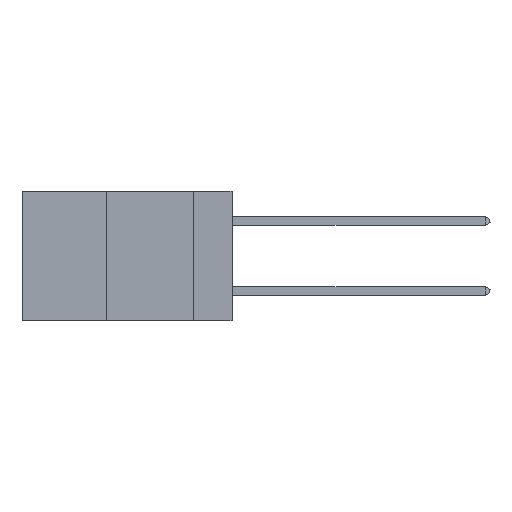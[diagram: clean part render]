
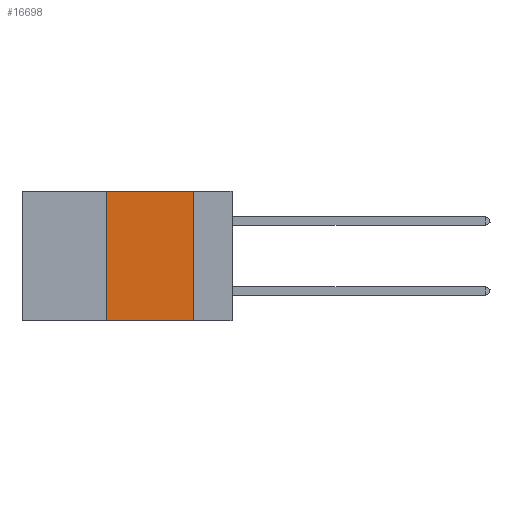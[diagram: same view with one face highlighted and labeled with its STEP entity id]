
A CAD part, left-side view. The second image highlights one B-rep face of the part: STEP entity #16698.
In plain terms, the highlighted planar face has unit normal (-1, 0, 0).
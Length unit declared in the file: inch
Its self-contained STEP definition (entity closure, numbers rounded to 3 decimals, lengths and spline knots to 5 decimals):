
#126 = VERTEX_POINT ( 'NONE', #13066 ) ;
#151 = LINE ( 'NONE', #2767, #1599 ) ;
#1599 = VECTOR ( 'NONE', #2745, 39.37008 ) ;
#2368 = VECTOR ( 'NONE', #10000, 39.37008 ) ;
#2745 = DIRECTION ( 'NONE',  ( 0., -1., 0. ) ) ;
#2767 = CARTESIAN_POINT ( 'NONE',  ( 0., 0.6, 0. ) ) ;
#3157 = CARTESIAN_POINT ( 'NONE',  ( 0., 0.36, 0. ) ) ;
#4890 = DIRECTION ( 'NONE',  ( 0., 0., -1. ) ) ;
#5109 = AXIS2_PLACEMENT_3D ( 'NONE', #5774, #8583, #13557 ) ;
#5685 = EDGE_CURVE ( 'NONE', #17000, #12538, #151, .T. ) ;
#5774 = CARTESIAN_POINT ( 'NONE',  ( 0., 0.6, 0. ) ) ;
#5812 = CARTESIAN_POINT ( 'NONE',  ( 0., 0.6, -0.37 ) ) ;
#5912 = ORIENTED_EDGE ( 'NONE', *, *, #5685, .F. ) ;
#6139 = LINE ( 'NONE', #5812, #2368 ) ;
#7488 = VERTEX_POINT ( 'NONE', #13101 ) ;
#7607 = LINE ( 'NONE', #10349, #17950 ) ;
#8424 = CARTESIAN_POINT ( 'NONE',  ( 0., 0.11, 0. ) ) ;
#8583 = DIRECTION ( 'NONE',  ( 1., 0., 0. ) ) ;
#8735 = EDGE_CURVE ( 'NONE', #12538, #126, #7607, .T. ) ;
#8835 = DIRECTION ( 'NONE',  ( 0., 0., 1. ) ) ;
#9533 = EDGE_LOOP ( 'NONE', ( #15918, #5912, #13139, #16035 ) ) ;
#9678 = LINE ( 'NONE', #3157, #15607 ) ;
#10000 = DIRECTION ( 'NONE',  ( 0., -1., 0. ) ) ;
#10349 = CARTESIAN_POINT ( 'NONE',  ( 0., 0.11, 0. ) ) ;
#10872 = EDGE_CURVE ( 'NONE', #7488, #17000, #9678, .T. ) ;
#12104 = FACE_OUTER_BOUND ( 'NONE', #9533, .T. ) ;
#12143 = CARTESIAN_POINT ( 'NONE',  ( 0., 0.36, 0. ) ) ;
#12538 = VERTEX_POINT ( 'NONE', #8424 ) ;
#13066 = CARTESIAN_POINT ( 'NONE',  ( 0., 0.11, -0.37 ) ) ;
#13101 = CARTESIAN_POINT ( 'NONE',  ( 0., 0.36, -0.37 ) ) ;
#13139 = ORIENTED_EDGE ( 'NONE', *, *, #10872, .F. ) ;
#13557 = DIRECTION ( 'NONE',  ( 0., 0., -1. ) ) ;
#15455 = EDGE_CURVE ( 'NONE', #7488, #126, #6139, .T. ) ;
#15607 = VECTOR ( 'NONE', #8835, 39.37008 ) ;
#15918 = ORIENTED_EDGE ( 'NONE', *, *, #8735, .F. ) ;
#16035 = ORIENTED_EDGE ( 'NONE', *, *, #15455, .T. ) ;
#16654 = PLANE ( 'NONE',  #5109 ) ;
#16698 = ADVANCED_FACE ( 'NONE', ( #12104 ), #16654, .F. ) ;
#17000 = VERTEX_POINT ( 'NONE', #12143 ) ;
#17950 = VECTOR ( 'NONE', #4890, 39.37008 ) ;
